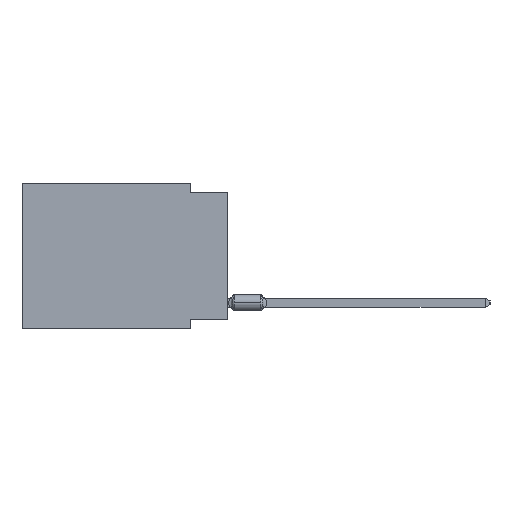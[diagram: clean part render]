
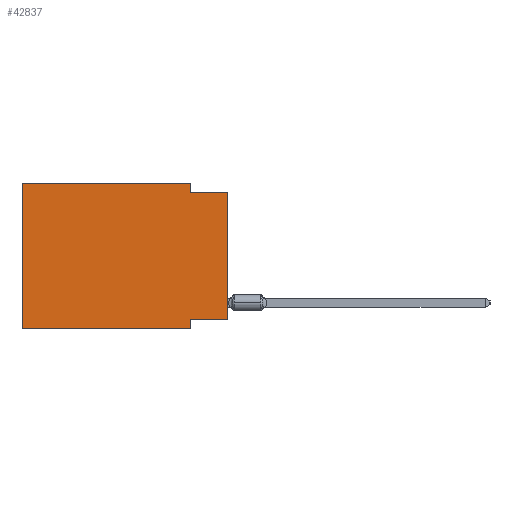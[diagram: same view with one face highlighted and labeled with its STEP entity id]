
A CAD part, left-side view. The second image highlights one B-rep face of the part: STEP entity #42837.
In plain terms, the highlighted planar face has unit normal (-1, 0, 0).
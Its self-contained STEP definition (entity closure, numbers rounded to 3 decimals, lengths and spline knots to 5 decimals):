
#1702 = EDGE_CURVE ( 'NONE', #15384, #68291, #3358, .T. ) ;
#3358 = LINE ( 'NONE', #84908, #42883 ) ;
#4126 = PLANE ( 'NONE',  #67450 ) ;
#4179 = DIRECTION ( 'NONE',  ( 0., -1., 0. ) ) ;
#4558 = DIRECTION ( 'NONE',  ( 0., 0., -1. ) ) ;
#4783 = ORIENTED_EDGE ( 'NONE', *, *, #14143, .F. ) ;
#11632 = VERTEX_POINT ( 'NONE', #21015 ) ;
#13915 = DIRECTION ( 'NONE',  ( 0., 0., -1. ) ) ;
#14143 = EDGE_CURVE ( 'NONE', #79625, #11632, #53616, .T. ) ;
#14625 = ORIENTED_EDGE ( 'NONE', *, *, #56342, .F. ) ;
#15384 = VERTEX_POINT ( 'NONE', #46944 ) ;
#15731 = EDGE_CURVE ( 'NONE', #34300, #34341, #17896, .T. ) ;
#16183 = CARTESIAN_POINT ( 'NONE',  ( 0., 0., 0. ) ) ;
#17182 = DIRECTION ( 'NONE',  ( 0., 1., 0. ) ) ;
#17896 = LINE ( 'NONE', #79824, #37240 ) ;
#18834 = CARTESIAN_POINT ( 'NONE',  ( 0., 0.1, 0. ) ) ;
#19915 = CARTESIAN_POINT ( 'NONE',  ( 0., 0.1, 0. ) ) ;
#19997 = CARTESIAN_POINT ( 'NONE',  ( 0., 0.1, -0.365 ) ) ;
#21015 = CARTESIAN_POINT ( 'NONE',  ( 0., 0., -0.025 ) ) ;
#21187 = VECTOR ( 'NONE', #57527, 39.37008 ) ;
#21696 = EDGE_CURVE ( 'NONE', #64365, #79625, #73631, .T. ) ;
#23538 = ORIENTED_EDGE ( 'NONE', *, *, #70281, .F. ) ;
#25596 = LINE ( 'NONE', #74162, #29040 ) ;
#25839 = VERTEX_POINT ( 'NONE', #69797 ) ;
#26679 = CARTESIAN_POINT ( 'NONE',  ( 0., 0.55, 0. ) ) ;
#26780 = EDGE_CURVE ( 'NONE', #68291, #34341, #51713, .T. ) ;
#28046 = CARTESIAN_POINT ( 'NONE',  ( 0., 0.1, -0.39 ) ) ;
#29040 = VECTOR ( 'NONE', #46074, 39.37008 ) ;
#29227 = ORIENTED_EDGE ( 'NONE', *, *, #21696, .F. ) ;
#31332 = ORIENTED_EDGE ( 'NONE', *, *, #1702, .F. ) ;
#31733 = VECTOR ( 'NONE', #52207, 39.37008 ) ;
#34300 = VERTEX_POINT ( 'NONE', #87317 ) ;
#34341 = VERTEX_POINT ( 'NONE', #28046 ) ;
#36339 = EDGE_LOOP ( 'NONE', ( #76845, #4783, #29227, #23538, #14625, #42174, #60640, #31332 ) ) ;
#36828 = EDGE_CURVE ( 'NONE', #15384, #11632, #77222, .T. ) ;
#37240 = VECTOR ( 'NONE', #38363, 39.37008 ) ;
#38363 = DIRECTION ( 'NONE',  ( 0., -1., 0. ) ) ;
#39827 = VECTOR ( 'NONE', #4179, 39.37008 ) ;
#42174 = ORIENTED_EDGE ( 'NONE', *, *, #15731, .T. ) ;
#42837 = ADVANCED_FACE ( 'NONE', ( #66051 ), #4126, .F. ) ;
#42883 = VECTOR ( 'NONE', #17182, 39.37008 ) ;
#43774 = DIRECTION ( 'NONE',  ( 0., 0., 1. ) ) ;
#46074 = DIRECTION ( 'NONE',  ( 0., -1., 0. ) ) ;
#46475 = CARTESIAN_POINT ( 'NONE',  ( 0., 0., -0.025 ) ) ;
#46944 = CARTESIAN_POINT ( 'NONE',  ( 0., 0., -0.365 ) ) ;
#51713 = LINE ( 'NONE', #78898, #21187 ) ;
#52207 = DIRECTION ( 'NONE',  ( 0., 0., 1. ) ) ;
#53616 = LINE ( 'NONE', #46475, #39827 ) ;
#56342 = EDGE_CURVE ( 'NONE', #34300, #25839, #86082, .T. ) ;
#57527 = DIRECTION ( 'NONE',  ( 0., 0., -1. ) ) ;
#60558 = VECTOR ( 'NONE', #13915, 39.37008 ) ;
#60640 = ORIENTED_EDGE ( 'NONE', *, *, #26780, .F. ) ;
#61047 = VECTOR ( 'NONE', #43774, 39.37008 ) ;
#64365 = VERTEX_POINT ( 'NONE', #19915 ) ;
#66051 = FACE_OUTER_BOUND ( 'NONE', #36339, .T. ) ;
#67450 = AXIS2_PLACEMENT_3D ( 'NONE', #78994, #71428, #4558 ) ;
#68291 = VERTEX_POINT ( 'NONE', #19997 ) ;
#69797 = CARTESIAN_POINT ( 'NONE',  ( 0., 0.55, 0. ) ) ;
#70074 = CARTESIAN_POINT ( 'NONE',  ( 0., 0.1, -0.025 ) ) ;
#70281 = EDGE_CURVE ( 'NONE', #25839, #64365, #25596, .T. ) ;
#71428 = DIRECTION ( 'NONE',  ( 1., 0., 0. ) ) ;
#73631 = LINE ( 'NONE', #18834, #60558 ) ;
#74162 = CARTESIAN_POINT ( 'NONE',  ( 0., 0.55, 0. ) ) ;
#76845 = ORIENTED_EDGE ( 'NONE', *, *, #36828, .T. ) ;
#77222 = LINE ( 'NONE', #16183, #61047 ) ;
#78898 = CARTESIAN_POINT ( 'NONE',  ( 0., 0.1, -0.39 ) ) ;
#78994 = CARTESIAN_POINT ( 'NONE',  ( 0., 0.55, 0. ) ) ;
#79625 = VERTEX_POINT ( 'NONE', #70074 ) ;
#79824 = CARTESIAN_POINT ( 'NONE',  ( 0., 0.55, -0.39 ) ) ;
#84908 = CARTESIAN_POINT ( 'NONE',  ( 0., 0., -0.365 ) ) ;
#86082 = LINE ( 'NONE', #26679, #31733 ) ;
#87317 = CARTESIAN_POINT ( 'NONE',  ( 0., 0.55, -0.39 ) ) ;
